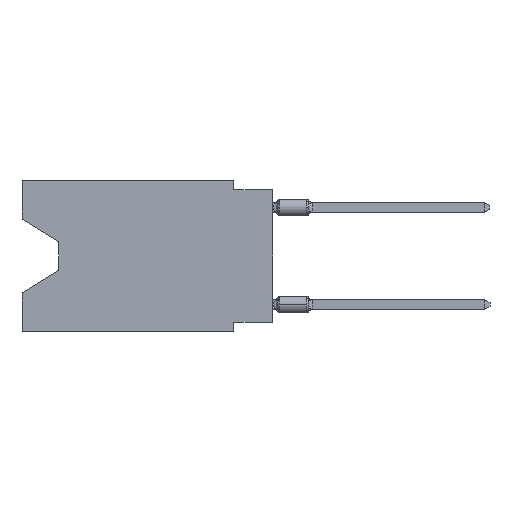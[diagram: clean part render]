
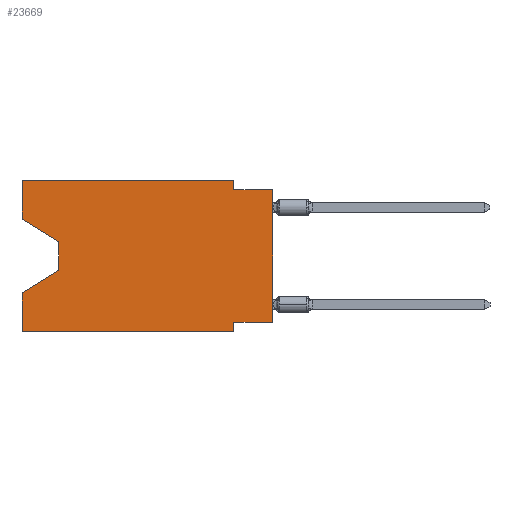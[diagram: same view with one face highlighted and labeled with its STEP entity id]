
A CAD part, left-side view. The second image highlights one B-rep face of the part: STEP entity #23669.
In plain terms, the highlighted planar face has unit normal (-1, 0, 0).
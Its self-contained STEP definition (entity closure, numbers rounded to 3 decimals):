
#275 = EDGE_CURVE ( 'NONE', #19247, #24953, #14278, .T. ) ;
#1173 = EDGE_CURVE ( 'NONE', #17739, #1582, #2514, .T. ) ;
#1222 = FACE_OUTER_BOUND ( 'NONE', #11597, .T. ) ;
#1415 = VERTEX_POINT ( 'NONE', #21159 ) ;
#1582 = VERTEX_POINT ( 'NONE', #26290 ) ;
#2198 = VECTOR ( 'NONE', #4872, 1000. ) ;
#2340 = LINE ( 'NONE', #8472, #8636 ) ;
#2514 = LINE ( 'NONE', #10406, #6153 ) ;
#3294 = LINE ( 'NONE', #23514, #15064 ) ;
#3398 = VECTOR ( 'NONE', #24178, 1000. ) ;
#4134 = VERTEX_POINT ( 'NONE', #8802 ) ;
#4435 = CARTESIAN_POINT ( 'NONE',  ( 0., 2.54, -9.271 ) ) ;
#4797 = ORIENTED_EDGE ( 'NONE', *, *, #22034, .T. ) ;
#4872 = DIRECTION ( 'NONE',  ( 0., 0., -1. ) ) ;
#5337 = CARTESIAN_POINT ( 'NONE',  ( 0., 2.54, -9.906 ) ) ;
#5340 = CARTESIAN_POINT ( 'NONE',  ( 0., 0., 0. ) ) ;
#5609 = DIRECTION ( 'NONE',  ( 0., 1., 0. ) ) ;
#6153 = VECTOR ( 'NONE', #25040, 1000. ) ;
#6165 = EDGE_CURVE ( 'NONE', #19562, #1415, #15686, .T. ) ;
#6551 = CARTESIAN_POINT ( 'NONE',  ( 0., 13.97, -5.893 ) ) ;
#8472 = CARTESIAN_POINT ( 'NONE',  ( 0., 16.383, 0. ) ) ;
#8636 = VECTOR ( 'NONE', #10506, 1000. ) ;
#8668 = EDGE_CURVE ( 'NONE', #16335, #1415, #16124, .T. ) ;
#8756 = VECTOR ( 'NONE', #20870, 1000. ) ;
#8802 = CARTESIAN_POINT ( 'NONE',  ( 0., 13.97, -4.013 ) ) ;
#9041 = ORIENTED_EDGE ( 'NONE', *, *, #14390, .T. ) ;
#9237 = EDGE_CURVE ( 'NONE', #21469, #19014, #15567, .T. ) ;
#9284 = EDGE_CURVE ( 'NONE', #11856, #24953, #16220, .T. ) ;
#9519 = CARTESIAN_POINT ( 'NONE',  ( 0., 16.383, 0. ) ) ;
#9674 = DIRECTION ( 'NONE',  ( 0., 0., 1. ) ) ;
#9837 = EDGE_CURVE ( 'NONE', #1582, #14700, #2340, .T. ) ;
#10004 = CARTESIAN_POINT ( 'NONE',  ( 0., 0., -9.271 ) ) ;
#10406 = CARTESIAN_POINT ( 'NONE',  ( 0., 16.383, 0. ) ) ;
#10506 = DIRECTION ( 'NONE',  ( 0., -1., 0. ) ) ;
#10981 = LINE ( 'NONE', #11513, #2198 ) ;
#11513 = CARTESIAN_POINT ( 'NONE',  ( 0., 2.54, 0. ) ) ;
#11597 = EDGE_LOOP ( 'NONE', ( #18477, #4797, #26191, #26219, #9041, #23619, #26665, #26487, #18463, #14099, #18841, #13475 ) ) ;
#11856 = VERTEX_POINT ( 'NONE', #12291 ) ;
#12115 = CARTESIAN_POINT ( 'NONE',  ( 0., 16.383, 0. ) ) ;
#12247 = DIRECTION ( 'NONE',  ( 0., 0., 1. ) ) ;
#12291 = CARTESIAN_POINT ( 'NONE',  ( 0., 16.383, -9.906 ) ) ;
#12900 = VECTOR ( 'NONE', #24601, 1000. ) ;
#12957 = CARTESIAN_POINT ( 'NONE',  ( 0., 2.54, 0. ) ) ;
#13062 = DIRECTION ( 'NONE',  ( 1., 0., 0. ) ) ;
#13098 = EDGE_CURVE ( 'NONE', #14700, #16335, #10981, .T. ) ;
#13399 = AXIS2_PLACEMENT_3D ( 'NONE', #9519, #13062, #23613 ) ;
#13475 = ORIENTED_EDGE ( 'NONE', *, *, #1173, .F. ) ;
#14099 = ORIENTED_EDGE ( 'NONE', *, *, #13098, .F. ) ;
#14278 = LINE ( 'NONE', #22503, #8756 ) ;
#14390 = EDGE_CURVE ( 'NONE', #11856, #19014, #21787, .T. ) ;
#14697 = VECTOR ( 'NONE', #12247, 1000. ) ;
#14700 = VERTEX_POINT ( 'NONE', #12957 ) ;
#14841 = CARTESIAN_POINT ( 'NONE',  ( 0., 16.383, -2.546 ) ) ;
#15064 = VECTOR ( 'NONE', #21458, 1000. ) ;
#15567 = LINE ( 'NONE', #21866, #3398 ) ;
#15623 = DIRECTION ( 'NONE',  ( 0., -1., 0. ) ) ;
#15686 = LINE ( 'NONE', #5340, #15888 ) ;
#15888 = VECTOR ( 'NONE', #9674, 1000. ) ;
#15996 = CARTESIAN_POINT ( 'NONE',  ( 0., 0., -0.635 ) ) ;
#16124 = LINE ( 'NONE', #15996, #18619 ) ;
#16220 = LINE ( 'NONE', #12115, #14697 ) ;
#16335 = VERTEX_POINT ( 'NONE', #19550 ) ;
#17739 = VERTEX_POINT ( 'NONE', #14841 ) ;
#17934 = VECTOR ( 'NONE', #15623, 1000. ) ;
#18015 = LINE ( 'NONE', #18276, #21638 ) ;
#18044 = DIRECTION ( 'NONE',  ( 0., -1., 0. ) ) ;
#18276 = CARTESIAN_POINT ( 'NONE',  ( 0., 0., -9.271 ) ) ;
#18463 = ORIENTED_EDGE ( 'NONE', *, *, #8668, .F. ) ;
#18477 = ORIENTED_EDGE ( 'NONE', *, *, #21667, .T. ) ;
#18619 = VECTOR ( 'NONE', #18044, 1000. ) ;
#18841 = ORIENTED_EDGE ( 'NONE', *, *, #9837, .F. ) ;
#19014 = VERTEX_POINT ( 'NONE', #5337 ) ;
#19247 = VERTEX_POINT ( 'NONE', #6551 ) ;
#19550 = CARTESIAN_POINT ( 'NONE',  ( 0., 2.54, -0.635 ) ) ;
#19562 = VERTEX_POINT ( 'NONE', #10004 ) ;
#19754 = PLANE ( 'NONE',  #13399 ) ;
#20506 = CARTESIAN_POINT ( 'NONE',  ( 0., 16.383, -2.546 ) ) ;
#20870 = DIRECTION ( 'NONE',  ( 0., 0.855, -0.519 ) ) ;
#21159 = CARTESIAN_POINT ( 'NONE',  ( 0., 0., -0.635 ) ) ;
#21279 = CARTESIAN_POINT ( 'NONE',  ( 0., 16.383, -7.36 ) ) ;
#21458 = DIRECTION ( 'NONE',  ( 0., 0., -1. ) ) ;
#21469 = VERTEX_POINT ( 'NONE', #4435 ) ;
#21638 = VECTOR ( 'NONE', #5609, 1000. ) ;
#21667 = EDGE_CURVE ( 'NONE', #17739, #4134, #25869, .T. ) ;
#21787 = LINE ( 'NONE', #26169, #17934 ) ;
#21866 = CARTESIAN_POINT ( 'NONE',  ( 0., 2.54, -9.906 ) ) ;
#22034 = EDGE_CURVE ( 'NONE', #4134, #19247, #3294, .T. ) ;
#22140 = EDGE_CURVE ( 'NONE', #19562, #21469, #18015, .T. ) ;
#22503 = CARTESIAN_POINT ( 'NONE',  ( 0., 13.97, -5.893 ) ) ;
#23514 = CARTESIAN_POINT ( 'NONE',  ( 0., 13.97, -4.013 ) ) ;
#23613 = DIRECTION ( 'NONE',  ( 0., 0., -1. ) ) ;
#23619 = ORIENTED_EDGE ( 'NONE', *, *, #9237, .F. ) ;
#23669 = ADVANCED_FACE ( 'NONE', ( #1222 ), #19754, .F. ) ;
#24178 = DIRECTION ( 'NONE',  ( 0., 0., -1. ) ) ;
#24601 = DIRECTION ( 'NONE',  ( 0., -0.855, -0.519 ) ) ;
#24953 = VERTEX_POINT ( 'NONE', #21279 ) ;
#25040 = DIRECTION ( 'NONE',  ( 0., 0., 1. ) ) ;
#25869 = LINE ( 'NONE', #20506, #12900 ) ;
#26169 = CARTESIAN_POINT ( 'NONE',  ( 0., 16.383, -9.906 ) ) ;
#26191 = ORIENTED_EDGE ( 'NONE', *, *, #275, .T. ) ;
#26219 = ORIENTED_EDGE ( 'NONE', *, *, #9284, .F. ) ;
#26290 = CARTESIAN_POINT ( 'NONE',  ( 0., 16.383, 0. ) ) ;
#26487 = ORIENTED_EDGE ( 'NONE', *, *, #6165, .T. ) ;
#26665 = ORIENTED_EDGE ( 'NONE', *, *, #22140, .F. ) ;
